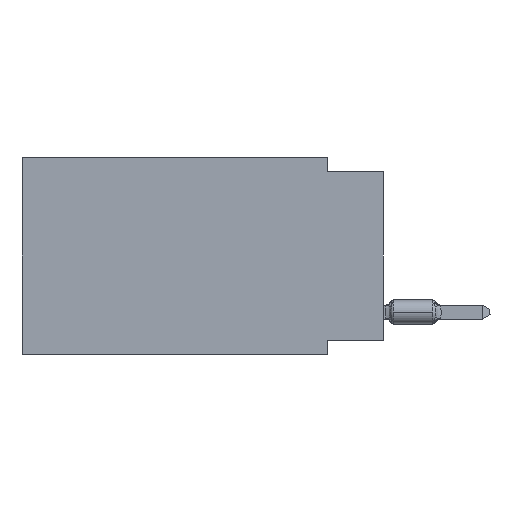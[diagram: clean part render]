
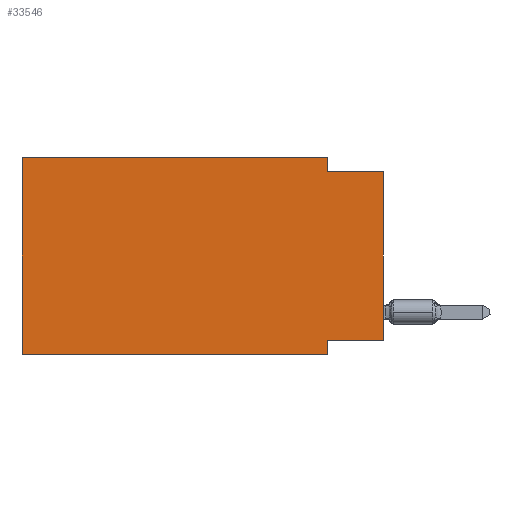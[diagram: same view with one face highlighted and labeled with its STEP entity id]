
A CAD part, left-side view. The second image highlights one B-rep face of the part: STEP entity #33546.
In plain terms, the highlighted planar face has unit normal (-1, 0, 0).
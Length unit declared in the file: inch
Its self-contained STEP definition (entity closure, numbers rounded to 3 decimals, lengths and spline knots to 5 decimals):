
#507 = CARTESIAN_POINT ( 'NONE',  ( 0., 0.1, -0.325 ) ) ;
#1454 = CARTESIAN_POINT ( 'NONE',  ( 0., 0.645, -0.35 ) ) ;
#1841 = AXIS2_PLACEMENT_3D ( 'NONE', #7074, #22914, #36137 ) ;
#2011 = DIRECTION ( 'NONE',  ( 0., 1., 0. ) ) ;
#2100 = CARTESIAN_POINT ( 'NONE',  ( 0., 0., -0.025 ) ) ;
#2443 = LINE ( 'NONE', #5659, #16892 ) ;
#2794 = DIRECTION ( 'NONE',  ( 0., 0., 1. ) ) ;
#2969 = PLANE ( 'NONE',  #1841 ) ;
#3260 = VERTEX_POINT ( 'NONE', #507 ) ;
#3390 = EDGE_CURVE ( 'NONE', #3260, #6141, #24308, .T. ) ;
#3617 = FACE_OUTER_BOUND ( 'NONE', #15943, .T. ) ;
#5659 = CARTESIAN_POINT ( 'NONE',  ( 0., 0., -0.325 ) ) ;
#6141 = VERTEX_POINT ( 'NONE', #32594 ) ;
#6675 = LINE ( 'NONE', #32515, #20385 ) ;
#6874 = EDGE_CURVE ( 'NONE', #29453, #27247, #18567, .T. ) ;
#6882 = ORIENTED_EDGE ( 'NONE', *, *, #38923, .F. ) ;
#7074 = CARTESIAN_POINT ( 'NONE',  ( 0., 0.645, 0. ) ) ;
#8302 = EDGE_CURVE ( 'NONE', #42580, #6141, #11852, .T. ) ;
#8980 = CARTESIAN_POINT ( 'NONE',  ( 0., 0., -0.025 ) ) ;
#11149 = DIRECTION ( 'NONE',  ( 0., 0., -1. ) ) ;
#11382 = VECTOR ( 'NONE', #12784, 39.37008 ) ;
#11411 = ORIENTED_EDGE ( 'NONE', *, *, #30268, .F. ) ;
#11852 = LINE ( 'NONE', #1454, #35187 ) ;
#12284 = CARTESIAN_POINT ( 'NONE',  ( 0., 0., -0.325 ) ) ;
#12784 = DIRECTION ( 'NONE',  ( 0., 0., 1. ) ) ;
#12992 = CARTESIAN_POINT ( 'NONE',  ( 0., 0.645, 0. ) ) ;
#15943 = EDGE_LOOP ( 'NONE', ( #38682, #40131, #41278, #11411, #20937, #20887, #22779, #6882 ) ) ;
#16517 = VECTOR ( 'NONE', #18458, 39.37008 ) ;
#16588 = VERTEX_POINT ( 'NONE', #30396 ) ;
#16892 = VECTOR ( 'NONE', #2011, 39.37008 ) ;
#18178 = DIRECTION ( 'NONE',  ( 0., -1., 0. ) ) ;
#18458 = DIRECTION ( 'NONE',  ( 0., 0., -1. ) ) ;
#18567 = LINE ( 'NONE', #2100, #34165 ) ;
#18580 = DIRECTION ( 'NONE',  ( 0., -1., 0. ) ) ;
#20385 = VECTOR ( 'NONE', #2794, 39.37008 ) ;
#20887 = ORIENTED_EDGE ( 'NONE', *, *, #8302, .T. ) ;
#20937 = ORIENTED_EDGE ( 'NONE', *, *, #31371, .F. ) ;
#21554 = LINE ( 'NONE', #24837, #37583 ) ;
#22225 = EDGE_CURVE ( 'NONE', #16588, #29453, #21554, .T. ) ;
#22767 = LINE ( 'NONE', #12992, #11382 ) ;
#22779 = ORIENTED_EDGE ( 'NONE', *, *, #3390, .F. ) ;
#22914 = DIRECTION ( 'NONE',  ( 1., 0., 0. ) ) ;
#24308 = LINE ( 'NONE', #31258, #16517 ) ;
#24658 = CARTESIAN_POINT ( 'NONE',  ( 0., 0.1, -0.025 ) ) ;
#24837 = CARTESIAN_POINT ( 'NONE',  ( 0., 0.1, 0. ) ) ;
#26573 = EDGE_CURVE ( 'NONE', #30773, #27247, #6675, .T. ) ;
#27247 = VERTEX_POINT ( 'NONE', #8980 ) ;
#28681 = VECTOR ( 'NONE', #18178, 39.37008 ) ;
#29453 = VERTEX_POINT ( 'NONE', #24658 ) ;
#29666 = CARTESIAN_POINT ( 'NONE',  ( 0., 0.645, 0. ) ) ;
#30268 = EDGE_CURVE ( 'NONE', #40382, #16588, #37731, .T. ) ;
#30396 = CARTESIAN_POINT ( 'NONE',  ( 0., 0.1, 0. ) ) ;
#30773 = VERTEX_POINT ( 'NONE', #12284 ) ;
#31258 = CARTESIAN_POINT ( 'NONE',  ( 0., 0.1, -0.35 ) ) ;
#31371 = EDGE_CURVE ( 'NONE', #42580, #40382, #22767, .T. ) ;
#31813 = DIRECTION ( 'NONE',  ( 0., -1., 0. ) ) ;
#32515 = CARTESIAN_POINT ( 'NONE',  ( 0., 0., 0. ) ) ;
#32594 = CARTESIAN_POINT ( 'NONE',  ( 0., 0.1, -0.35 ) ) ;
#33546 = ADVANCED_FACE ( 'NONE', ( #3617 ), #2969, .F. ) ;
#34165 = VECTOR ( 'NONE', #31813, 39.37008 ) ;
#35187 = VECTOR ( 'NONE', #18580, 39.37008 ) ;
#36137 = DIRECTION ( 'NONE',  ( 0., 0., -1. ) ) ;
#37583 = VECTOR ( 'NONE', #11149, 39.37008 ) ;
#37731 = LINE ( 'NONE', #39982, #28681 ) ;
#38682 = ORIENTED_EDGE ( 'NONE', *, *, #26573, .T. ) ;
#38923 = EDGE_CURVE ( 'NONE', #30773, #3260, #2443, .T. ) ;
#39982 = CARTESIAN_POINT ( 'NONE',  ( 0., 0.645, 0. ) ) ;
#40131 = ORIENTED_EDGE ( 'NONE', *, *, #6874, .F. ) ;
#40382 = VERTEX_POINT ( 'NONE', #29666 ) ;
#40599 = CARTESIAN_POINT ( 'NONE',  ( 0., 0.645, -0.35 ) ) ;
#41278 = ORIENTED_EDGE ( 'NONE', *, *, #22225, .F. ) ;
#42580 = VERTEX_POINT ( 'NONE', #40599 ) ;
